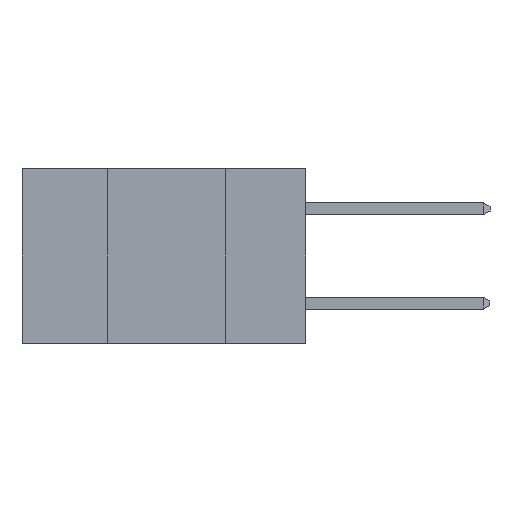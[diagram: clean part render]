
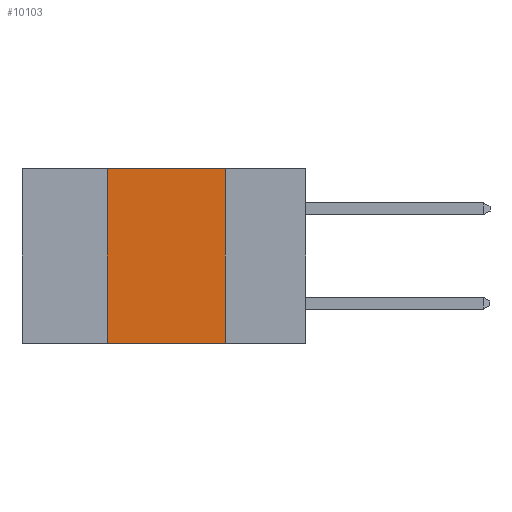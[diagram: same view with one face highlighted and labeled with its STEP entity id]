
A CAD part, left-side view. The second image highlights one B-rep face of the part: STEP entity #10103.
In plain terms, the highlighted planar face has unit normal (-1, 0, 0).
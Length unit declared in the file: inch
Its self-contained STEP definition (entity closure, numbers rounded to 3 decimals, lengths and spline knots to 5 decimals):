
#23 = CARTESIAN_POINT ( 'NONE',  ( 0., 0.42, 0. ) ) ;
#271 = CARTESIAN_POINT ( 'NONE',  ( 0., 0.17, 0. ) ) ;
#802 = LINE ( 'NONE', #1689, #10584 ) ;
#1636 = VECTOR ( 'NONE', #15704, 39.37008 ) ;
#1689 = CARTESIAN_POINT ( 'NONE',  ( 0., 0.6, -0.37 ) ) ;
#1743 = DIRECTION ( 'NONE',  ( 0., -1., 0. ) ) ;
#1994 = LINE ( 'NONE', #271, #12142 ) ;
#2882 = ORIENTED_EDGE ( 'NONE', *, *, #4115, .T. ) ;
#4115 = EDGE_CURVE ( 'NONE', #7511, #6005, #802, .T. ) ;
#4955 = LINE ( 'NONE', #10401, #1636 ) ;
#5198 = VERTEX_POINT ( 'NONE', #23 ) ;
#5393 = LINE ( 'NONE', #11291, #8461 ) ;
#5425 = CARTESIAN_POINT ( 'NONE',  ( 0., 0.17, -0.37 ) ) ;
#5675 = CARTESIAN_POINT ( 'NONE',  ( 0., 0.6, 0. ) ) ;
#5693 = CARTESIAN_POINT ( 'NONE',  ( 0., 0.42, -0.37 ) ) ;
#6005 = VERTEX_POINT ( 'NONE', #5425 ) ;
#6672 = FACE_OUTER_BOUND ( 'NONE', #7981, .T. ) ;
#6982 = DIRECTION ( 'NONE',  ( 1., 0., 0. ) ) ;
#7511 = VERTEX_POINT ( 'NONE', #5693 ) ;
#7746 = EDGE_CURVE ( 'NONE', #7511, #5198, #5393, .T. ) ;
#7913 = DIRECTION ( 'NONE',  ( 0., 0., -1. ) ) ;
#7981 = EDGE_LOOP ( 'NONE', ( #12515, #14452, #11651, #2882 ) ) ;
#8324 = CARTESIAN_POINT ( 'NONE',  ( 0., 0.17, 0. ) ) ;
#8461 = VECTOR ( 'NONE', #12582, 39.37008 ) ;
#8679 = EDGE_CURVE ( 'NONE', #5198, #13852, #4955, .T. ) ;
#10103 = ADVANCED_FACE ( 'NONE', ( #6672 ), #13369, .F. ) ;
#10195 = AXIS2_PLACEMENT_3D ( 'NONE', #5675, #6982, #15872 ) ;
#10401 = CARTESIAN_POINT ( 'NONE',  ( 0., 0.6, 0. ) ) ;
#10584 = VECTOR ( 'NONE', #1743, 39.37008 ) ;
#11291 = CARTESIAN_POINT ( 'NONE',  ( 0., 0.42, 0. ) ) ;
#11651 = ORIENTED_EDGE ( 'NONE', *, *, #7746, .F. ) ;
#12142 = VECTOR ( 'NONE', #7913, 39.37008 ) ;
#12515 = ORIENTED_EDGE ( 'NONE', *, *, #14174, .F. ) ;
#12582 = DIRECTION ( 'NONE',  ( 0., 0., 1. ) ) ;
#13369 = PLANE ( 'NONE',  #10195 ) ;
#13852 = VERTEX_POINT ( 'NONE', #8324 ) ;
#14174 = EDGE_CURVE ( 'NONE', #13852, #6005, #1994, .T. ) ;
#14452 = ORIENTED_EDGE ( 'NONE', *, *, #8679, .F. ) ;
#15704 = DIRECTION ( 'NONE',  ( 0., -1., 0. ) ) ;
#15872 = DIRECTION ( 'NONE',  ( 0., 0., -1. ) ) ;
